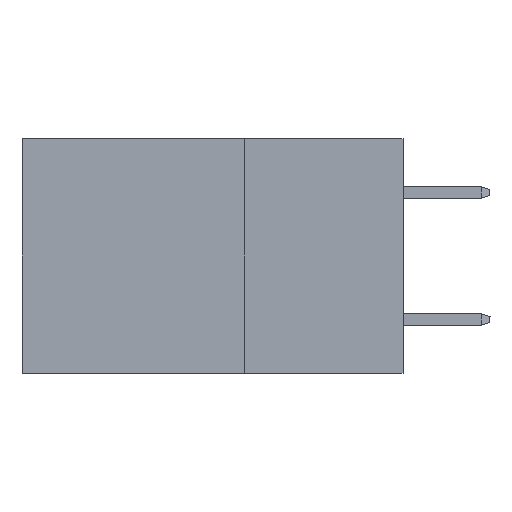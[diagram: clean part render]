
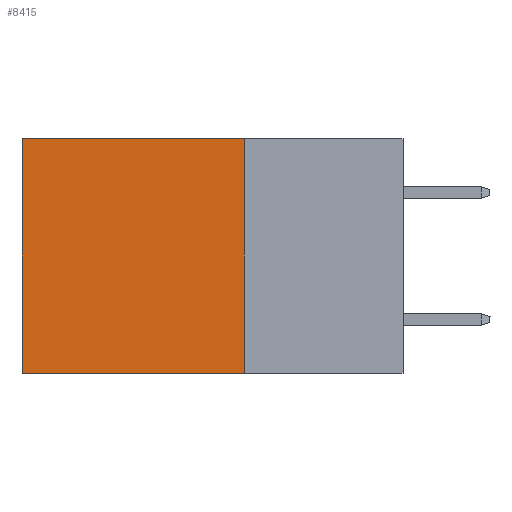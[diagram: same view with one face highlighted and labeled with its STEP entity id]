
A CAD part, left-side view. The second image highlights one B-rep face of the part: STEP entity #8415.
In plain terms, the highlighted planar face has unit normal (-1, 0, 0).
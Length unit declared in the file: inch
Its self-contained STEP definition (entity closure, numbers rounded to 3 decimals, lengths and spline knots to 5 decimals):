
#128 = CARTESIAN_POINT ( 'NONE',  ( 0.2875, 0.6, 0. ) ) ;
#503 = DIRECTION ( 'NONE',  ( 0., 0., -1. ) ) ;
#2020 = CARTESIAN_POINT ( 'NONE',  ( 0.2875, 0.25, -0.37 ) ) ;
#3635 = PLANE ( 'NONE',  #8427 ) ;
#4052 = CARTESIAN_POINT ( 'NONE',  ( 0.2875, 0.25, 0. ) ) ;
#5895 = CARTESIAN_POINT ( 'NONE',  ( 0.2875, 0.6, 0. ) ) ;
#6155 = LINE ( 'NONE', #7569, #10774 ) ;
#6162 = VERTEX_POINT ( 'NONE', #19743 ) ;
#6271 = EDGE_CURVE ( 'NONE', #21074, #18915, #6155, .T. ) ;
#7135 = ORIENTED_EDGE ( 'NONE', *, *, #13360, .T. ) ;
#7298 = DIRECTION ( 'NONE',  ( 1., 0., 0. ) ) ;
#7568 = DIRECTION ( 'NONE',  ( 0., 0., -1. ) ) ;
#7569 = CARTESIAN_POINT ( 'NONE',  ( 0.2875, 0.25, -0.37 ) ) ;
#7796 = LINE ( 'NONE', #128, #20104 ) ;
#8415 = ADVANCED_FACE ( 'NONE', ( #10523 ), #3635, .F. ) ;
#8427 = AXIS2_PLACEMENT_3D ( 'NONE', #9088, #7298, #21675 ) ;
#9088 = CARTESIAN_POINT ( 'NONE',  ( 0.2875, 0.25, 0. ) ) ;
#10512 = DIRECTION ( 'NONE',  ( 0., 1., 0. ) ) ;
#10523 = FACE_OUTER_BOUND ( 'NONE', #17352, .T. ) ;
#10667 = VERTEX_POINT ( 'NONE', #5895 ) ;
#10774 = VECTOR ( 'NONE', #15241, 39.37008 ) ;
#11695 = EDGE_CURVE ( 'NONE', #6162, #21074, #13025, .T. ) ;
#13025 = LINE ( 'NONE', #4052, #14044 ) ;
#13360 = EDGE_CURVE ( 'NONE', #10667, #18915, #7796, .T. ) ;
#13662 = ORIENTED_EDGE ( 'NONE', *, *, #6271, .F. ) ;
#14044 = VECTOR ( 'NONE', #503, 39.37008 ) ;
#14612 = EDGE_CURVE ( 'NONE', #6162, #10667, #21207, .T. ) ;
#15241 = DIRECTION ( 'NONE',  ( 0., 1., 0. ) ) ;
#17352 = EDGE_LOOP ( 'NONE', ( #7135, #13662, #19980, #22867 ) ) ;
#18915 = VERTEX_POINT ( 'NONE', #21406 ) ;
#19451 = CARTESIAN_POINT ( 'NONE',  ( 0.2875, 0.25, 0. ) ) ;
#19743 = CARTESIAN_POINT ( 'NONE',  ( 0.2875, 0.25, 0. ) ) ;
#19980 = ORIENTED_EDGE ( 'NONE', *, *, #11695, .F. ) ;
#20104 = VECTOR ( 'NONE', #7568, 39.37008 ) ;
#21074 = VERTEX_POINT ( 'NONE', #2020 ) ;
#21207 = LINE ( 'NONE', #19451, #21660 ) ;
#21406 = CARTESIAN_POINT ( 'NONE',  ( 0.2875, 0.6, -0.37 ) ) ;
#21660 = VECTOR ( 'NONE', #10512, 39.37008 ) ;
#21675 = DIRECTION ( 'NONE',  ( 0., 0., -1. ) ) ;
#22867 = ORIENTED_EDGE ( 'NONE', *, *, #14612, .T. ) ;
